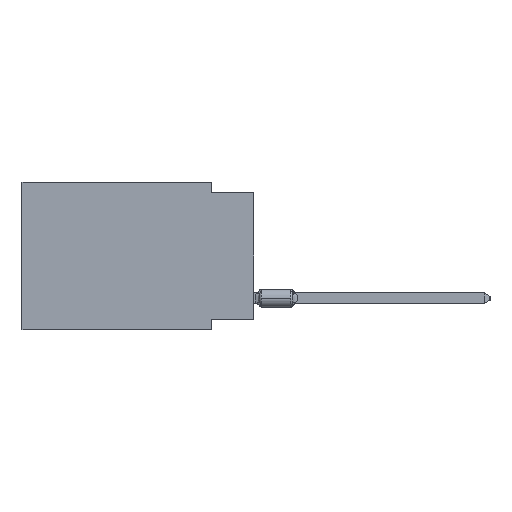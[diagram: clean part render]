
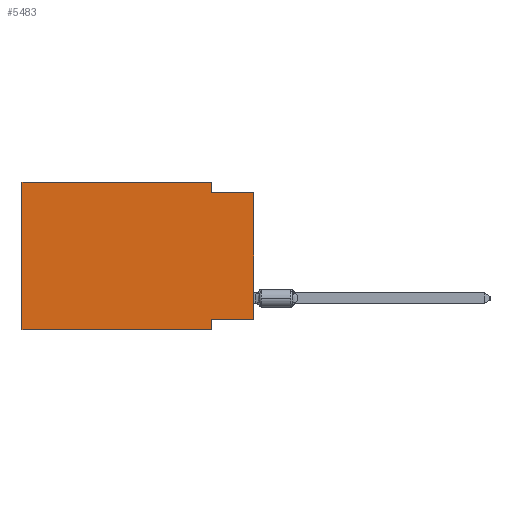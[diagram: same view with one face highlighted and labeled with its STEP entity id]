
A CAD part, left-side view. The second image highlights one B-rep face of the part: STEP entity #5483.
In plain terms, the highlighted planar face has unit normal (-1, 0, 0).
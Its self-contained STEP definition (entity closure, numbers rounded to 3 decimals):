
#457 = VERTEX_POINT ( 'NONE', #47820 ) ;
#1078 = ORIENTED_EDGE ( 'NONE', *, *, #6023, .F. ) ;
#1120 = VERTEX_POINT ( 'NONE', #45652 ) ;
#2167 = ORIENTED_EDGE ( 'NONE', *, *, #15305, .T. ) ;
#2468 = EDGE_CURVE ( 'NONE', #1120, #5743, #38452, .T. ) ;
#2524 = DIRECTION ( 'NONE',  ( 1., 0., 0. ) ) ;
#2562 = LINE ( 'NONE', #45659, #43756 ) ;
#5483 = ADVANCED_FACE ( 'NONE', ( #37409 ), #29852, .F. ) ;
#5743 = VERTEX_POINT ( 'NONE', #9244 ) ;
#6023 = EDGE_CURVE ( 'NONE', #15773, #48558, #30309, .T. ) ;
#6057 = DIRECTION ( 'NONE',  ( 0., 1., 0. ) ) ;
#7190 = EDGE_CURVE ( 'NONE', #5743, #15773, #11154, .T. ) ;
#8597 = EDGE_CURVE ( 'NONE', #457, #22518, #32438, .T. ) ;
#8731 = ORIENTED_EDGE ( 'NONE', *, *, #29750, .F. ) ;
#9244 = CARTESIAN_POINT ( 'NONE',  ( 0., 13.97, 0. ) ) ;
#9836 = VERTEX_POINT ( 'NONE', #10200 ) ;
#10200 = CARTESIAN_POINT ( 'NONE',  ( 0., 0., -8.255 ) ) ;
#11154 = LINE ( 'NONE', #41522, #15847 ) ;
#11647 = DIRECTION ( 'NONE',  ( 0., -1., 0. ) ) ;
#12743 = EDGE_LOOP ( 'NONE', ( #37137, #19951, #1078, #35039, #36660, #2167, #27155, #8731 ) ) ;
#14476 = CARTESIAN_POINT ( 'NONE',  ( 0., 2.54, 0. ) ) ;
#15305 = EDGE_CURVE ( 'NONE', #1120, #22518, #2562, .T. ) ;
#15773 = VERTEX_POINT ( 'NONE', #14476 ) ;
#15847 = VECTOR ( 'NONE', #11647, 1000. ) ;
#16030 = VECTOR ( 'NONE', #33524, 1000. ) ;
#17941 = VERTEX_POINT ( 'NONE', #48508 ) ;
#18509 = EDGE_CURVE ( 'NONE', #48558, #17941, #41018, .T. ) ;
#19951 = ORIENTED_EDGE ( 'NONE', *, *, #18509, .F. ) ;
#22518 = VERTEX_POINT ( 'NONE', #42648 ) ;
#22768 = CARTESIAN_POINT ( 'NONE',  ( 0., 0., 0. ) ) ;
#23805 = AXIS2_PLACEMENT_3D ( 'NONE', #44922, #2524, #37652 ) ;
#25109 = CARTESIAN_POINT ( 'NONE',  ( 0., 0., -8.255 ) ) ;
#26530 = CARTESIAN_POINT ( 'NONE',  ( 0., 2.54, 0. ) ) ;
#26882 = DIRECTION ( 'NONE',  ( 0., 0., 1. ) ) ;
#27155 = ORIENTED_EDGE ( 'NONE', *, *, #8597, .F. ) ;
#29459 = VECTOR ( 'NONE', #45619, 1000. ) ;
#29750 = EDGE_CURVE ( 'NONE', #9836, #457, #40683, .T. ) ;
#29852 = PLANE ( 'NONE',  #23805 ) ;
#30309 = LINE ( 'NONE', #26530, #29459 ) ;
#30310 = LINE ( 'NONE', #22768, #45200 ) ;
#30718 = CARTESIAN_POINT ( 'NONE',  ( 0., 0., -0.635 ) ) ;
#32438 = LINE ( 'NONE', #39989, #42387 ) ;
#33524 = DIRECTION ( 'NONE',  ( 0., -1., 0. ) ) ;
#35039 = ORIENTED_EDGE ( 'NONE', *, *, #7190, .F. ) ;
#35267 = VECTOR ( 'NONE', #26882, 1000. ) ;
#36660 = ORIENTED_EDGE ( 'NONE', *, *, #2468, .F. ) ;
#37137 = ORIENTED_EDGE ( 'NONE', *, *, #41145, .T. ) ;
#37409 = FACE_OUTER_BOUND ( 'NONE', #12743, .T. ) ;
#37652 = DIRECTION ( 'NONE',  ( 0., 0., -1. ) ) ;
#37865 = DIRECTION ( 'NONE',  ( 0., -1., 0. ) ) ;
#38049 = CARTESIAN_POINT ( 'NONE',  ( 0., 2.54, -0.635 ) ) ;
#38452 = LINE ( 'NONE', #49230, #35267 ) ;
#39989 = CARTESIAN_POINT ( 'NONE',  ( 0., 2.54, -8.89 ) ) ;
#40683 = LINE ( 'NONE', #25109, #44489 ) ;
#41018 = LINE ( 'NONE', #30718, #16030 ) ;
#41145 = EDGE_CURVE ( 'NONE', #9836, #17941, #30310, .T. ) ;
#41522 = CARTESIAN_POINT ( 'NONE',  ( 0., 13.97, 0. ) ) ;
#42359 = DIRECTION ( 'NONE',  ( 0., 0., 1. ) ) ;
#42387 = VECTOR ( 'NONE', #47764, 1000. ) ;
#42648 = CARTESIAN_POINT ( 'NONE',  ( 0., 2.54, -8.89 ) ) ;
#43756 = VECTOR ( 'NONE', #37865, 1000. ) ;
#44489 = VECTOR ( 'NONE', #6057, 1000. ) ;
#44922 = CARTESIAN_POINT ( 'NONE',  ( 0., 13.97, 0. ) ) ;
#45200 = VECTOR ( 'NONE', #42359, 1000. ) ;
#45619 = DIRECTION ( 'NONE',  ( 0., 0., -1. ) ) ;
#45652 = CARTESIAN_POINT ( 'NONE',  ( 0., 13.97, -8.89 ) ) ;
#45659 = CARTESIAN_POINT ( 'NONE',  ( 0., 13.97, -8.89 ) ) ;
#47764 = DIRECTION ( 'NONE',  ( 0., 0., -1. ) ) ;
#47820 = CARTESIAN_POINT ( 'NONE',  ( 0., 2.54, -8.255 ) ) ;
#48508 = CARTESIAN_POINT ( 'NONE',  ( 0., 0., -0.635 ) ) ;
#48558 = VERTEX_POINT ( 'NONE', #38049 ) ;
#49230 = CARTESIAN_POINT ( 'NONE',  ( 0., 13.97, 0. ) ) ;
